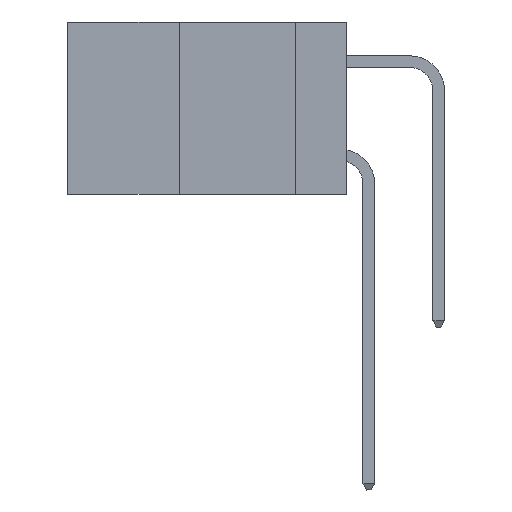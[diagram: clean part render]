
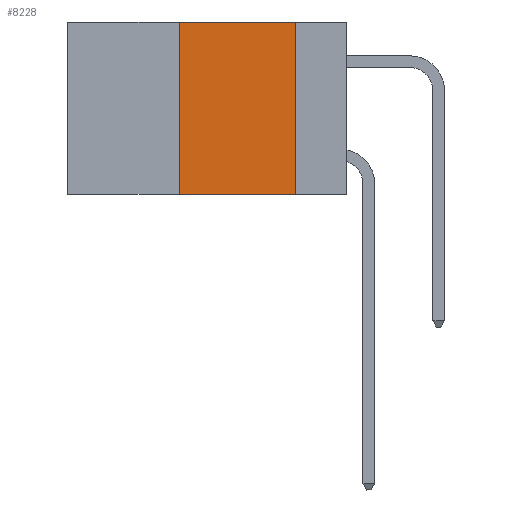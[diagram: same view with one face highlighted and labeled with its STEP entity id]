
A CAD part, left-side view. The second image highlights one B-rep face of the part: STEP entity #8228.
In plain terms, the highlighted planar face has unit normal (-1, 0, 0).
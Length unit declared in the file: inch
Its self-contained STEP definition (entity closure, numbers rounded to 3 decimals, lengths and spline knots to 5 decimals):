
#210 = ORIENTED_EDGE ( 'NONE', *, *, #7185, .T. ) ;
#272 = DIRECTION ( 'NONE',  ( 0., 0., -1. ) ) ;
#1240 = LINE ( 'NONE', #2957, #14467 ) ;
#1446 = CARTESIAN_POINT ( 'NONE',  ( 0., 0.6, 0. ) ) ;
#2957 = CARTESIAN_POINT ( 'NONE',  ( 0., 0.36, 0. ) ) ;
#3390 = EDGE_CURVE ( 'NONE', #10300, #6938, #1240, .T. ) ;
#3425 = AXIS2_PLACEMENT_3D ( 'NONE', #1446, #13130, #272 ) ;
#3565 = DIRECTION ( 'NONE',  ( 0., -1., 0. ) ) ;
#4762 = EDGE_CURVE ( 'NONE', #6938, #15213, #13230, .T. ) ;
#6242 = CARTESIAN_POINT ( 'NONE',  ( 0., 0.11, 0. ) ) ;
#6343 = FACE_OUTER_BOUND ( 'NONE', #11115, .T. ) ;
#6427 = CARTESIAN_POINT ( 'NONE',  ( 0., 0.11, 0. ) ) ;
#6938 = VERTEX_POINT ( 'NONE', #11403 ) ;
#7185 = EDGE_CURVE ( 'NONE', #10300, #10052, #13579, .T. ) ;
#7719 = CARTESIAN_POINT ( 'NONE',  ( 0., 0.11, -0.37 ) ) ;
#8228 = ADVANCED_FACE ( 'NONE', ( #6343 ), #13071, .F. ) ;
#8386 = VECTOR ( 'NONE', #10340, 39.37008 ) ;
#8430 = VECTOR ( 'NONE', #3565, 39.37008 ) ;
#10052 = VERTEX_POINT ( 'NONE', #7719 ) ;
#10217 = CARTESIAN_POINT ( 'NONE',  ( 0., 0.6, 0. ) ) ;
#10281 = ORIENTED_EDGE ( 'NONE', *, *, #15205, .F. ) ;
#10300 = VERTEX_POINT ( 'NONE', #10471 ) ;
#10340 = DIRECTION ( 'NONE',  ( 0., -1., 0. ) ) ;
#10471 = CARTESIAN_POINT ( 'NONE',  ( 0., 0.36, -0.37 ) ) ;
#10843 = DIRECTION ( 'NONE',  ( 0., 0., 1. ) ) ;
#11115 = EDGE_LOOP ( 'NONE', ( #10281, #15628, #11596, #210 ) ) ;
#11403 = CARTESIAN_POINT ( 'NONE',  ( 0., 0.36, 0. ) ) ;
#11596 = ORIENTED_EDGE ( 'NONE', *, *, #3390, .F. ) ;
#12049 = VECTOR ( 'NONE', #15324, 39.37008 ) ;
#12836 = CARTESIAN_POINT ( 'NONE',  ( 0., 0.6, -0.37 ) ) ;
#13071 = PLANE ( 'NONE',  #3425 ) ;
#13130 = DIRECTION ( 'NONE',  ( 1., 0., 0. ) ) ;
#13230 = LINE ( 'NONE', #10217, #8430 ) ;
#13579 = LINE ( 'NONE', #12836, #8386 ) ;
#13643 = LINE ( 'NONE', #6427, #12049 ) ;
#14467 = VECTOR ( 'NONE', #10843, 39.37008 ) ;
#15205 = EDGE_CURVE ( 'NONE', #15213, #10052, #13643, .T. ) ;
#15213 = VERTEX_POINT ( 'NONE', #6242 ) ;
#15324 = DIRECTION ( 'NONE',  ( 0., 0., -1. ) ) ;
#15628 = ORIENTED_EDGE ( 'NONE', *, *, #4762, .F. ) ;
